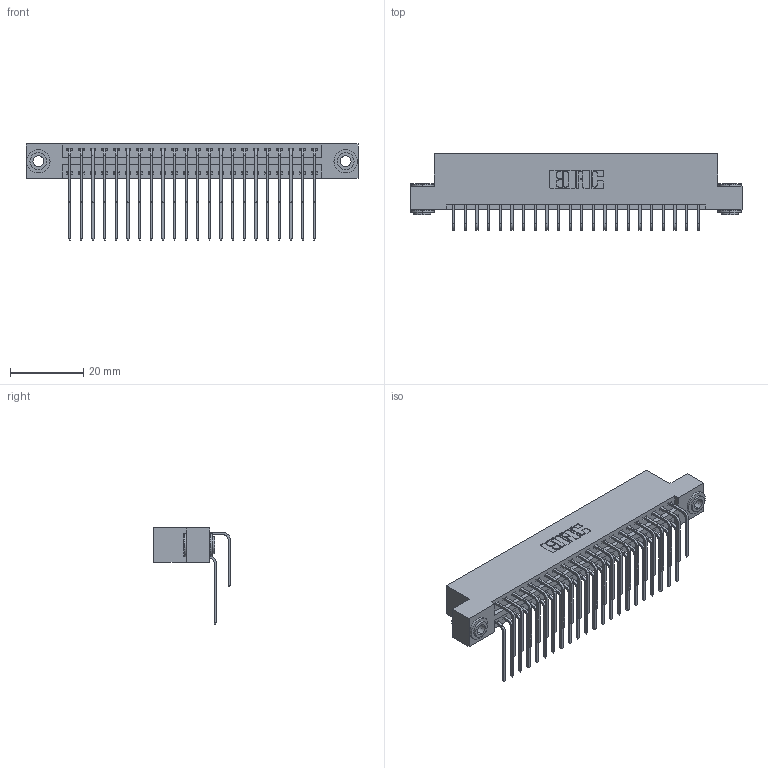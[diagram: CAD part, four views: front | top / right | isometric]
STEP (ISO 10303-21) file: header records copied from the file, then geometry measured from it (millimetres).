
FILE_DESCRIPTION (( 'STEP AP203' ), '1' );
FILE_NAME ('396-044-559-203.STEP', '2019-11-03T07:57:02', ( '' ), ( '' ), 'SwSTEP 2.0', 'SolidWorks 2016', '' );
FILE_SCHEMA (( 'CONFIG_CONTROL_DESIGN' ));
Length unit declared in the file: inch
Products named in the file (5): 345-250-002_345-250-002-102; 345-292-001_559 Tail - 2; 346 Part_Flush Mounting Lugs - 0.156 Dia-TH; 396-044-559-203; 345-292-001_558 559 Tail - 1
Assembly tree (47 placements, depth 2):
  396-044-559-203
    346 Part_Flush Mounting Lugs - 0.156 Dia-TH
    345-292-001_558 559 Tail - 1  x22
    345-292-001_559 Tail - 2  x22
    345-250-002_345-250-002-102  x2
Bounding box: 90.42 x 20.89 x 26.16 mm (x, y, z)
Volume: 8935.3 mm3; surface area: 13399.7 mm2
Topology: 47 solids, 47 shells, 2536 faces, 7489 edges, 4930 vertices
Faces by surface type: plane 1714, cylinder 814, cone 8
Entity records: 19484 total; most frequent: CARTESIAN_POINT 3266, ORIENTED_EDGE 3142, DIRECTION 2933, EDGE_CURVE 1571, LINE 1287, VECTOR 1287, VERTEX_POINT 1042, AXIS2_PLACEMENT_3D 823
